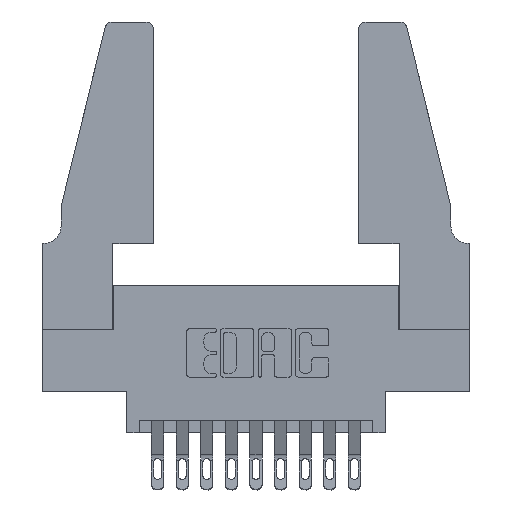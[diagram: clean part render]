
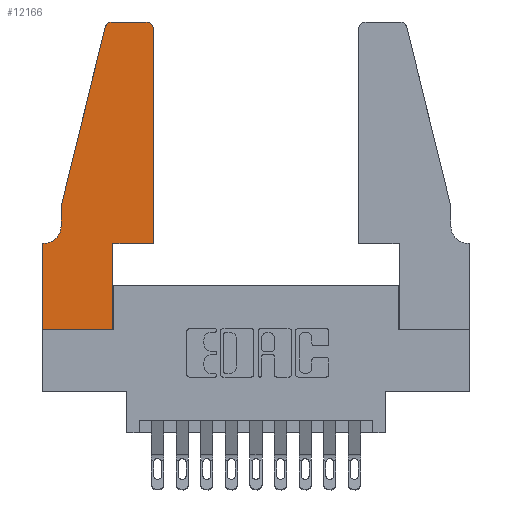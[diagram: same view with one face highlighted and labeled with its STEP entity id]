
A CAD part, top view. The second image highlights one B-rep face of the part: STEP entity #12166.
In plain terms, the highlighted planar face has unit normal (0, 0, 1).
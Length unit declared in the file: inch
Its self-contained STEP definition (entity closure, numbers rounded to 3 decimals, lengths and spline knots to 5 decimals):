
#95 = VERTEX_POINT ( 'NONE', #11146 ) ;
#110 = LINE ( 'NONE', #4446, #4808 ) ;
#272 = VECTOR ( 'NONE', #12732, 39.37008 ) ;
#391 = DIRECTION ( 'NONE',  ( 0., 0., 1. ) ) ;
#431 = CARTESIAN_POINT ( 'NONE',  ( 0.284, 1.22, 0.37 ) ) ;
#529 = CARTESIAN_POINT ( 'NONE',  ( 0.0755, 0.42, 0.37 ) ) ;
#599 = CARTESIAN_POINT ( 'NONE',  ( 0.4505, 0.35, 0.37 ) ) ;
#715 = ORIENTED_EDGE ( 'NONE', *, *, #7030, .T. ) ;
#721 = EDGE_CURVE ( 'NONE', #3147, #5567, #9941, .T. ) ;
#736 = ORIENTED_EDGE ( 'NONE', *, *, #2344, .T. ) ;
#748 = VERTEX_POINT ( 'NONE', #2024 ) ;
#876 = FACE_OUTER_BOUND ( 'NONE', #9793, .T. ) ;
#1011 = VECTOR ( 'NONE', #1818, 39.37008 ) ;
#1450 = ORIENTED_EDGE ( 'NONE', *, *, #9795, .T. ) ;
#1465 = VERTEX_POINT ( 'NONE', #4758 ) ;
#1602 = DIRECTION ( 'NONE',  ( 1., 0., 0. ) ) ;
#1706 = CARTESIAN_POINT ( 'NONE',  ( 0.4205, 1.25, 0.37 ) ) ;
#1739 = CARTESIAN_POINT ( 'NONE',  ( 0.2605, 1.25, 0.37 ) ) ;
#1818 = DIRECTION ( 'NONE',  ( 0., 1., 0. ) ) ;
#1870 = CARTESIAN_POINT ( 'NONE',  ( 0.4505, 0.35, 0.37 ) ) ;
#1917 = CARTESIAN_POINT ( 'NONE',  ( 0., 0., 0.37 ) ) ;
#1948 = ORIENTED_EDGE ( 'NONE', *, *, #6105, .T. ) ;
#2024 = CARTESIAN_POINT ( 'NONE',  ( 0.25487, 1.22718, 0.37 ) ) ;
#2130 = CARTESIAN_POINT ( 'NONE',  ( 0., 0., 0.37 ) ) ;
#2276 = DIRECTION ( 'NONE',  ( 0., 0., 1. ) ) ;
#2305 = AXIS2_PLACEMENT_3D ( 'NONE', #2660, #10203, #3793 ) ;
#2344 = EDGE_CURVE ( 'NONE', #95, #4730, #8216, .T. ) ;
#2487 = CARTESIAN_POINT ( 'NONE',  ( 0.4505, 1.22, 0.37 ) ) ;
#2660 = CARTESIAN_POINT ( 'NONE',  ( 0.0055, 0.42, 0.37 ) ) ;
#2782 = AXIS2_PLACEMENT_3D ( 'NONE', #8791, #2276, #9868 ) ;
#2977 = ORIENTED_EDGE ( 'NONE', *, *, #8322, .T. ) ;
#3147 = VERTEX_POINT ( 'NONE', #1706 ) ;
#3355 = DIRECTION ( 'NONE',  ( -1., 0., 0. ) ) ;
#3599 = CIRCLE ( 'NONE', #2782, 0.03 ) ;
#3606 = DIRECTION ( 'NONE',  ( -1., 0., 0. ) ) ;
#3685 = VECTOR ( 'NONE', #9355, 39.37008 ) ;
#3793 = DIRECTION ( 'NONE',  ( -1., 0., 0. ) ) ;
#3851 = CARTESIAN_POINT ( 'NONE',  ( 0.0755, 0.35, 0.37 ) ) ;
#3888 = VERTEX_POINT ( 'NONE', #12388 ) ;
#4090 = LINE ( 'NONE', #599, #1011 ) ;
#4185 = VERTEX_POINT ( 'NONE', #4638 ) ;
#4251 = ORIENTED_EDGE ( 'NONE', *, *, #6584, .T. ) ;
#4321 = CARTESIAN_POINT ( 'NONE',  ( 0.0755, 0.5, 0.37 ) ) ;
#4446 = CARTESIAN_POINT ( 'NONE',  ( 0.0755, 0.5, 0.37 ) ) ;
#4568 = CARTESIAN_POINT ( 'NONE',  ( 0.284, 1.25, 0.37 ) ) ;
#4592 = AXIS2_PLACEMENT_3D ( 'NONE', #431, #8185, #1602 ) ;
#4638 = CARTESIAN_POINT ( 'NONE',  ( 0.0755, 0.5, 0.37 ) ) ;
#4685 = VERTEX_POINT ( 'NONE', #13236 ) ;
#4730 = VERTEX_POINT ( 'NONE', #10794 ) ;
#4758 = CARTESIAN_POINT ( 'NONE',  ( 0.2865, 0., 0.37 ) ) ;
#4799 = EDGE_CURVE ( 'NONE', #4730, #4685, #11802, .T. ) ;
#4808 = VECTOR ( 'NONE', #5562, 39.37008 ) ;
#5106 = AXIS2_PLACEMENT_3D ( 'NONE', #7104, #391, #8147 ) ;
#5291 = CIRCLE ( 'NONE', #4592, 0.03 ) ;
#5537 = EDGE_CURVE ( 'NONE', #8081, #3147, #3599, .T. ) ;
#5562 = DIRECTION ( 'NONE',  ( 0., -1., 0. ) ) ;
#5567 = VERTEX_POINT ( 'NONE', #4568 ) ;
#5897 = ORIENTED_EDGE ( 'NONE', *, *, #721, .T. ) ;
#6061 = PLANE ( 'NONE',  #5106 ) ;
#6105 = EDGE_CURVE ( 'NONE', #4185, #7192, #110, .T. ) ;
#6398 = ORIENTED_EDGE ( 'NONE', *, *, #6725, .T. ) ;
#6501 = VECTOR ( 'NONE', #8668, 39.37008 ) ;
#6584 = EDGE_CURVE ( 'NONE', #9069, #8081, #4090, .T. ) ;
#6634 = LINE ( 'NONE', #1917, #272 ) ;
#6640 = EDGE_CURVE ( 'NONE', #4685, #1465, #6634, .T. ) ;
#6725 = EDGE_CURVE ( 'NONE', #3888, #9069, #8428, .T. ) ;
#6994 = ORIENTED_EDGE ( 'NONE', *, *, #7106, .T. ) ;
#7030 = EDGE_CURVE ( 'NONE', #7192, #95, #9427, .T. ) ;
#7104 = CARTESIAN_POINT ( 'NONE',  ( 0., 0.35, 0.37 ) ) ;
#7106 = EDGE_CURVE ( 'NONE', #5567, #748, #5291, .T. ) ;
#7192 = VERTEX_POINT ( 'NONE', #529 ) ;
#7263 = CARTESIAN_POINT ( 'NONE',  ( 0.2865, 0.35, 0.37 ) ) ;
#7687 = LINE ( 'NONE', #4321, #10520 ) ;
#8081 = VERTEX_POINT ( 'NONE', #2487 ) ;
#8147 = DIRECTION ( 'NONE',  ( 1., 0., 0. ) ) ;
#8185 = DIRECTION ( 'NONE',  ( 0., 0., 1. ) ) ;
#8216 = LINE ( 'NONE', #3851, #13561 ) ;
#8322 = EDGE_CURVE ( 'NONE', #1465, #3888, #12228, .T. ) ;
#8428 = LINE ( 'NONE', #10716, #13424 ) ;
#8668 = DIRECTION ( 'NONE',  ( 0., -1., 0. ) ) ;
#8791 = CARTESIAN_POINT ( 'NONE',  ( 0.4205, 1.22, 0.37 ) ) ;
#9069 = VERTEX_POINT ( 'NONE', #1870 ) ;
#9355 = DIRECTION ( 'NONE',  ( 0., 1., 0. ) ) ;
#9427 = CIRCLE ( 'NONE', #2305, 0.07 ) ;
#9634 = DIRECTION ( 'NONE',  ( -0.239, -0.971, 0. ) ) ;
#9793 = EDGE_LOOP ( 'NONE', ( #5897, #6994, #1450, #1948, #715, #736, #10653, #12710, #2977, #6398, #4251, #12591 ) ) ;
#9795 = EDGE_CURVE ( 'NONE', #748, #4185, #7687, .T. ) ;
#9868 = DIRECTION ( 'NONE',  ( 1., 0., 0. ) ) ;
#9941 = LINE ( 'NONE', #1739, #10269 ) ;
#10203 = DIRECTION ( 'NONE',  ( 0., 0., -1. ) ) ;
#10269 = VECTOR ( 'NONE', #3355, 39.37008 ) ;
#10520 = VECTOR ( 'NONE', #9634, 39.37008 ) ;
#10653 = ORIENTED_EDGE ( 'NONE', *, *, #4799, .T. ) ;
#10716 = CARTESIAN_POINT ( 'NONE',  ( 0.4505, 0.35, 0.37 ) ) ;
#10794 = CARTESIAN_POINT ( 'NONE',  ( 0., 0.35, 0.37 ) ) ;
#11146 = CARTESIAN_POINT ( 'NONE',  ( 0.0055, 0.35, 0.37 ) ) ;
#11802 = LINE ( 'NONE', #2130, #6501 ) ;
#12166 = ADVANCED_FACE ( 'NONE', ( #876 ), #6061, .T. ) ;
#12228 = LINE ( 'NONE', #7263, #3685 ) ;
#12388 = CARTESIAN_POINT ( 'NONE',  ( 0.2865, 0.35, 0.37 ) ) ;
#12591 = ORIENTED_EDGE ( 'NONE', *, *, #5537, .T. ) ;
#12710 = ORIENTED_EDGE ( 'NONE', *, *, #6640, .T. ) ;
#12732 = DIRECTION ( 'NONE',  ( 1., 0., 0. ) ) ;
#13236 = CARTESIAN_POINT ( 'NONE',  ( 0., 0., 0.37 ) ) ;
#13424 = VECTOR ( 'NONE', #13914, 39.37008 ) ;
#13561 = VECTOR ( 'NONE', #3606, 39.37008 ) ;
#13914 = DIRECTION ( 'NONE',  ( 1., 0., 0. ) ) ;
